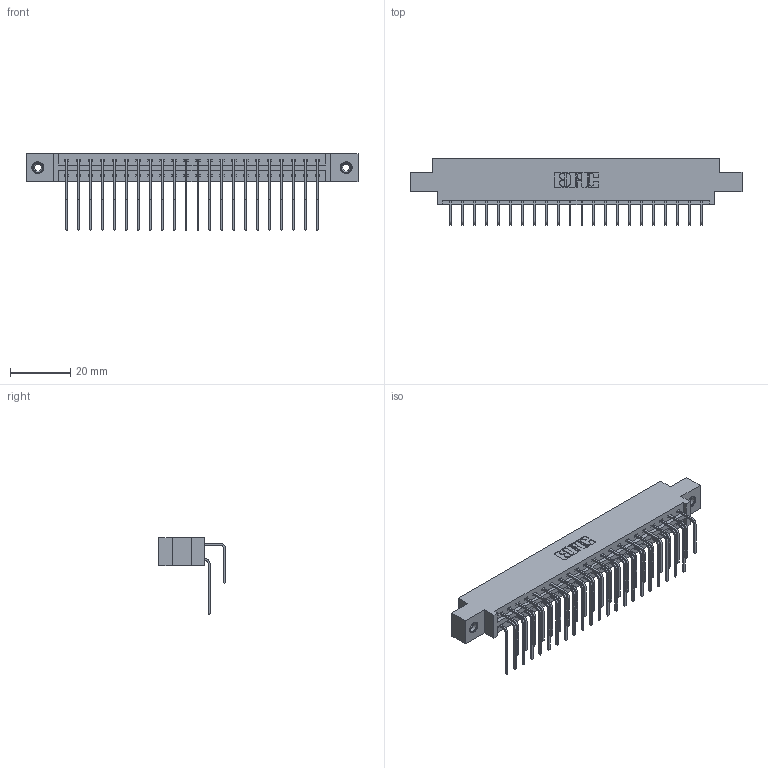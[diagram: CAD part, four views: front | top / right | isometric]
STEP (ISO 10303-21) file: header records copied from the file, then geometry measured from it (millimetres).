
FILE_DESCRIPTION (( 'STEP AP203' ), '1' );
FILE_NAME ('387-044-558-808.STEP', '2018-09-20T02:58:08', ( '' ), ( '' ), 'SwSTEP 2.0', 'SolidWorks 2016', '' );
FILE_SCHEMA (( 'CONFIG_CONTROL_DESIGN' ));
Length unit declared in the file: inch
Products named in the file (5): 337 Part_0.170 Offset - 0.156 Dia-TI; 345-292-001_558 559 Tail - 1; 345-292-001_558 Tail - 2; 345-250-001_345-250-003-102; 387-044-558-808
Assembly tree (47 placements, depth 2):
  387-044-558-808
    337 Part_0.170 Offset - 0.156 Dia-TI
    345-292-001_558 559 Tail - 1  x22
    345-292-001_558 Tail - 2  x22
    345-250-001_345-250-003-102  x2
Bounding box: 110.19 x 22.17 x 25.53 mm (x, y, z)
Volume: 11475.8 mm3; surface area: 14185.4 mm2
Topology: 47 solids, 47 shells, 2642 faces, 7807 edges, 5138 vertices
Faces by surface type: plane 1866, cylinder 760, cone 12, torus 4
Entity records: 22746 total; most frequent: CARTESIAN_POINT 3876, ORIENTED_EDGE 3754, DIRECTION 3347, EDGE_CURVE 1877, LINE 1689, VECTOR 1689, VERTEX_POINT 1244, AXIS2_PLACEMENT_3D 829
